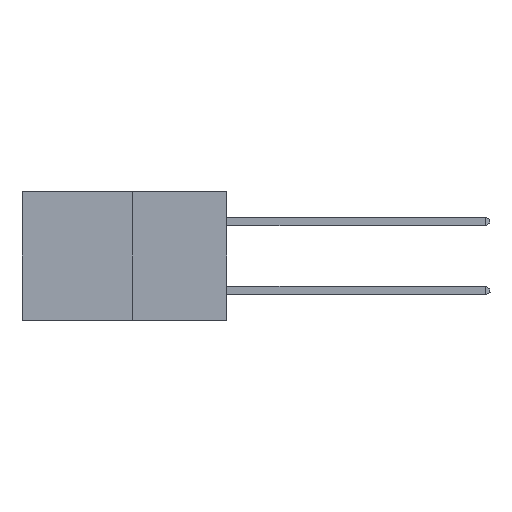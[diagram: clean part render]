
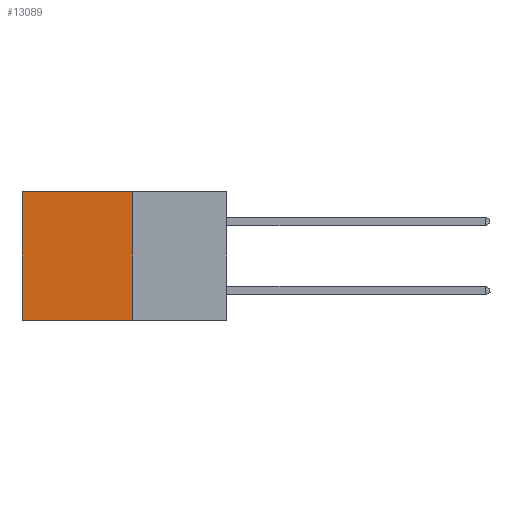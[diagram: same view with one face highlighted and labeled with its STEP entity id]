
A CAD part, left-side view. The second image highlights one B-rep face of the part: STEP entity #13089.
In plain terms, the highlighted planar face has unit normal (-1, 0, 0).
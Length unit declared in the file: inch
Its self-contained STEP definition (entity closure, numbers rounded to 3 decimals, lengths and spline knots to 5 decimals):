
#17 = CARTESIAN_POINT ( 'NONE',  ( 0.277, 0.59, -0.37 ) ) ;
#531 = VERTEX_POINT ( 'NONE', #10352 ) ;
#862 = AXIS2_PLACEMENT_3D ( 'NONE', #14425, #13298, #6173 ) ;
#928 = CARTESIAN_POINT ( 'NONE',  ( 0.277, 0.27, 0. ) ) ;
#1004 = LINE ( 'NONE', #928, #13032 ) ;
#1318 = EDGE_CURVE ( 'NONE', #13870, #5746, #11694, .T. ) ;
#1964 = CARTESIAN_POINT ( 'NONE',  ( 0.277, 0.27, -0.37 ) ) ;
#2699 = ORIENTED_EDGE ( 'NONE', *, *, #1318, .F. ) ;
#2981 = VERTEX_POINT ( 'NONE', #7861 ) ;
#3408 = DIRECTION ( 'NONE',  ( 0., 1., 0. ) ) ;
#4087 = EDGE_CURVE ( 'NONE', #531, #13870, #15410, .T. ) ;
#4103 = LINE ( 'NONE', #10130, #10038 ) ;
#5746 = VERTEX_POINT ( 'NONE', #17 ) ;
#6173 = DIRECTION ( 'NONE',  ( 0., 0., -1. ) ) ;
#6360 = VECTOR ( 'NONE', #10459, 39.37008 ) ;
#7861 = CARTESIAN_POINT ( 'NONE',  ( 0.277, 0.59, 0. ) ) ;
#8120 = VECTOR ( 'NONE', #9360, 39.37008 ) ;
#8259 = ORIENTED_EDGE ( 'NONE', *, *, #11142, .T. ) ;
#9360 = DIRECTION ( 'NONE',  ( 0., 1., 0. ) ) ;
#9446 = ORIENTED_EDGE ( 'NONE', *, *, #11350, .T. ) ;
#9832 = CARTESIAN_POINT ( 'NONE',  ( 0.277, 0.27, -0.37 ) ) ;
#10038 = VECTOR ( 'NONE', #11361, 39.37008 ) ;
#10082 = EDGE_LOOP ( 'NONE', ( #8259, #2699, #12784, #9446 ) ) ;
#10130 = CARTESIAN_POINT ( 'NONE',  ( 0.277, 0.59, -0.37 ) ) ;
#10352 = CARTESIAN_POINT ( 'NONE',  ( 0.277, 0.27, 0. ) ) ;
#10459 = DIRECTION ( 'NONE',  ( 0., 0., -1. ) ) ;
#10544 = FACE_OUTER_BOUND ( 'NONE', #10082, .T. ) ;
#11142 = EDGE_CURVE ( 'NONE', #2981, #5746, #4103, .T. ) ;
#11350 = EDGE_CURVE ( 'NONE', #531, #2981, #1004, .T. ) ;
#11361 = DIRECTION ( 'NONE',  ( 0., 0., -1. ) ) ;
#11503 = CARTESIAN_POINT ( 'NONE',  ( 0.277, 0.27, -0.37 ) ) ;
#11694 = LINE ( 'NONE', #11503, #8120 ) ;
#12128 = PLANE ( 'NONE',  #862 ) ;
#12784 = ORIENTED_EDGE ( 'NONE', *, *, #4087, .F. ) ;
#13032 = VECTOR ( 'NONE', #3408, 39.37008 ) ;
#13089 = ADVANCED_FACE ( 'NONE', ( #10544 ), #12128, .F. ) ;
#13298 = DIRECTION ( 'NONE',  ( 1., 0., 0. ) ) ;
#13870 = VERTEX_POINT ( 'NONE', #9832 ) ;
#14425 = CARTESIAN_POINT ( 'NONE',  ( 0.277, 0.27, -0.37 ) ) ;
#15410 = LINE ( 'NONE', #1964, #6360 ) ;
